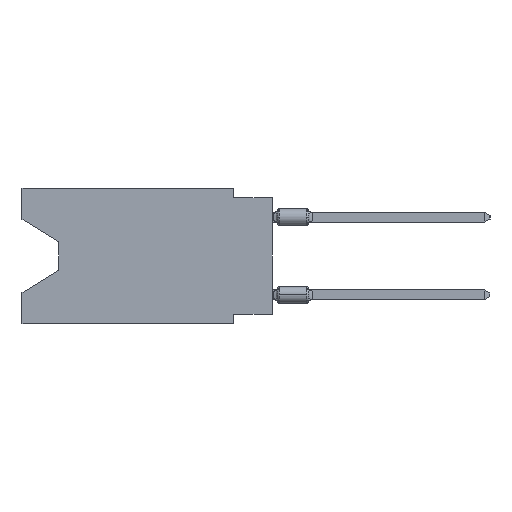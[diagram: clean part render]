
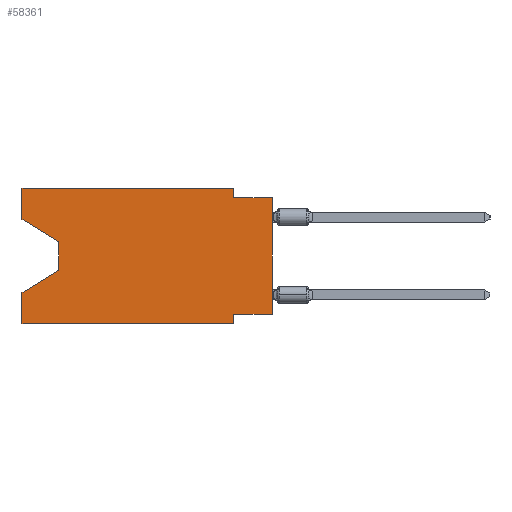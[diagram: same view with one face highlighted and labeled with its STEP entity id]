
A CAD part, left-side view. The second image highlights one B-rep face of the part: STEP entity #58361.
In plain terms, the highlighted planar face has unit normal (-1, 0, 0).
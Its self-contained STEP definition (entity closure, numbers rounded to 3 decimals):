
#2 = CARTESIAN_POINT ( 'NONE',  ( 0., 13.97, -5.385 ) ) ;
#44 = LINE ( 'NONE', #68377, #68410 ) ;
#96 = VERTEX_POINT ( 'NONE', #14504 ) ;
#595 = VERTEX_POINT ( 'NONE', #54141 ) ;
#1430 = ORIENTED_EDGE ( 'NONE', *, *, #9033, .T. ) ;
#1491 = EDGE_CURVE ( 'NONE', #27973, #48108, #33830, .T. ) ;
#1894 = LINE ( 'NONE', #55572, #65405 ) ;
#3446 = EDGE_CURVE ( 'NONE', #29089, #27973, #61913, .T. ) ;
#4562 = VECTOR ( 'NONE', #18804, 1000. ) ;
#4643 = DIRECTION ( 'NONE',  ( 0., 0., -1. ) ) ;
#6801 = CARTESIAN_POINT ( 'NONE',  ( 0., 2.54, 0. ) ) ;
#7218 = CARTESIAN_POINT ( 'NONE',  ( 0., 16.383, -2.038 ) ) ;
#8457 = VECTOR ( 'NONE', #26323, 1000. ) ;
#8740 = CARTESIAN_POINT ( 'NONE',  ( 0., 16.383, -6.852 ) ) ;
#9033 = EDGE_CURVE ( 'NONE', #48108, #32076, #20736, .T. ) ;
#9254 = CARTESIAN_POINT ( 'NONE',  ( 0., 0., -8.255 ) ) ;
#10105 = EDGE_CURVE ( 'NONE', #14759, #96, #62402, .T. ) ;
#11089 = ORIENTED_EDGE ( 'NONE', *, *, #20183, .T. ) ;
#11769 = ORIENTED_EDGE ( 'NONE', *, *, #59760, .F. ) ;
#12449 = DIRECTION ( 'NONE',  ( 0., -1., 0. ) ) ;
#12720 = AXIS2_PLACEMENT_3D ( 'NONE', #62862, #52406, #4643 ) ;
#12785 = CARTESIAN_POINT ( 'NONE',  ( 0., 13.97, -3.505 ) ) ;
#14504 = CARTESIAN_POINT ( 'NONE',  ( 0., 2.54, -8.89 ) ) ;
#14759 = VERTEX_POINT ( 'NONE', #41415 ) ;
#14832 = LINE ( 'NONE', #9254, #31881 ) ;
#18024 = EDGE_LOOP ( 'NONE', ( #64068, #19802, #1430, #45340, #11089, #64749, #50941, #44433, #61040, #11769, #22272, #67755 ) ) ;
#18804 = DIRECTION ( 'NONE',  ( 0., 0., -1. ) ) ;
#19235 = VECTOR ( 'NONE', #25319, 1000. ) ;
#19802 = ORIENTED_EDGE ( 'NONE', *, *, #1491, .T. ) ;
#20183 = EDGE_CURVE ( 'NONE', #51797, #96, #40516, .T. ) ;
#20736 = LINE ( 'NONE', #64302, #8457 ) ;
#20793 = VECTOR ( 'NONE', #41653, 1000. ) ;
#22272 = ORIENTED_EDGE ( 'NONE', *, *, #30496, .F. ) ;
#23642 = LINE ( 'NONE', #30855, #20793 ) ;
#25023 = EDGE_CURVE ( 'NONE', #51797, #32076, #55082, .T. ) ;
#25319 = DIRECTION ( 'NONE',  ( 0., -0.855, -0.519 ) ) ;
#25593 = FACE_OUTER_BOUND ( 'NONE', #18024, .T. ) ;
#26323 = DIRECTION ( 'NONE',  ( 0., 0.855, -0.519 ) ) ;
#26567 = DIRECTION ( 'NONE',  ( 0., 0., 1. ) ) ;
#26668 = VECTOR ( 'NONE', #28956, 1000. ) ;
#27403 = VERTEX_POINT ( 'NONE', #52255 ) ;
#27493 = CARTESIAN_POINT ( 'NONE',  ( 0., 0., -0.635 ) ) ;
#27973 = VERTEX_POINT ( 'NONE', #12785 ) ;
#28956 = DIRECTION ( 'NONE',  ( 0., 0., 1. ) ) ;
#29051 = EDGE_CURVE ( 'NONE', #27403, #51496, #37946, .T. ) ;
#29089 = VERTEX_POINT ( 'NONE', #7218 ) ;
#29853 = DIRECTION ( 'NONE',  ( 0., 1., 0. ) ) ;
#30100 = CARTESIAN_POINT ( 'NONE',  ( 0., 2.54, 0. ) ) ;
#30496 = EDGE_CURVE ( 'NONE', #34547, #38015, #1894, .T. ) ;
#30855 = CARTESIAN_POINT ( 'NONE',  ( 0., 16.383, 0. ) ) ;
#31881 = VECTOR ( 'NONE', #29853, 1000. ) ;
#32076 = VERTEX_POINT ( 'NONE', #8740 ) ;
#33830 = LINE ( 'NONE', #34517, #4562 ) ;
#34517 = CARTESIAN_POINT ( 'NONE',  ( 0., 13.97, -3.505 ) ) ;
#34547 = VERTEX_POINT ( 'NONE', #50335 ) ;
#35319 = EDGE_CURVE ( 'NONE', #595, #14759, #14832, .T. ) ;
#37768 = VECTOR ( 'NONE', #61787, 1000. ) ;
#37946 = LINE ( 'NONE', #27493, #57774 ) ;
#38015 = VERTEX_POINT ( 'NONE', #30100 ) ;
#40516 = LINE ( 'NONE', #66329, #37768 ) ;
#41415 = CARTESIAN_POINT ( 'NONE',  ( 0., 2.54, -8.255 ) ) ;
#41602 = PLANE ( 'NONE',  #12720 ) ;
#41653 = DIRECTION ( 'NONE',  ( 0., 0., 1. ) ) ;
#44433 = ORIENTED_EDGE ( 'NONE', *, *, #59942, .T. ) ;
#45301 = CARTESIAN_POINT ( 'NONE',  ( 0., 16.383, 0. ) ) ;
#45340 = ORIENTED_EDGE ( 'NONE', *, *, #25023, .F. ) ;
#47210 = VECTOR ( 'NONE', #54554, 1000. ) ;
#47427 = CARTESIAN_POINT ( 'NONE',  ( 0., 16.383, -8.89 ) ) ;
#48108 = VERTEX_POINT ( 'NONE', #2 ) ;
#50335 = CARTESIAN_POINT ( 'NONE',  ( 0., 16.383, 0. ) ) ;
#50941 = ORIENTED_EDGE ( 'NONE', *, *, #35319, .F. ) ;
#50961 = LINE ( 'NONE', #6801, #47210 ) ;
#51496 = VERTEX_POINT ( 'NONE', #54580 ) ;
#51797 = VERTEX_POINT ( 'NONE', #47427 ) ;
#52255 = CARTESIAN_POINT ( 'NONE',  ( 0., 2.54, -0.635 ) ) ;
#52281 = DIRECTION ( 'NONE',  ( 0., 0., -1. ) ) ;
#52406 = DIRECTION ( 'NONE',  ( 1., 0., 0. ) ) ;
#54141 = CARTESIAN_POINT ( 'NONE',  ( 0., 0., -8.255 ) ) ;
#54554 = DIRECTION ( 'NONE',  ( 0., 0., -1. ) ) ;
#54580 = CARTESIAN_POINT ( 'NONE',  ( 0., 0., -0.635 ) ) ;
#55082 = LINE ( 'NONE', #45301, #26668 ) ;
#55572 = CARTESIAN_POINT ( 'NONE',  ( 0., 16.383, 0. ) ) ;
#56735 = EDGE_CURVE ( 'NONE', #29089, #34547, #23642, .T. ) ;
#57015 = CARTESIAN_POINT ( 'NONE',  ( 0., 16.383, -2.038 ) ) ;
#57511 = CARTESIAN_POINT ( 'NONE',  ( 0., 2.54, -8.89 ) ) ;
#57774 = VECTOR ( 'NONE', #12449, 1000. ) ;
#58361 = ADVANCED_FACE ( 'NONE', ( #25593 ), #41602, .F. ) ;
#59760 = EDGE_CURVE ( 'NONE', #38015, #27403, #50961, .T. ) ;
#59942 = EDGE_CURVE ( 'NONE', #595, #51496, #44, .T. ) ;
#60482 = DIRECTION ( 'NONE',  ( 0., -1., 0. ) ) ;
#61040 = ORIENTED_EDGE ( 'NONE', *, *, #29051, .F. ) ;
#61787 = DIRECTION ( 'NONE',  ( 0., -1., 0. ) ) ;
#61913 = LINE ( 'NONE', #57015, #19235 ) ;
#62073 = VECTOR ( 'NONE', #52281, 1000. ) ;
#62402 = LINE ( 'NONE', #57511, #62073 ) ;
#62862 = CARTESIAN_POINT ( 'NONE',  ( 0., 16.383, 0. ) ) ;
#64068 = ORIENTED_EDGE ( 'NONE', *, *, #3446, .T. ) ;
#64302 = CARTESIAN_POINT ( 'NONE',  ( 0., 13.97, -5.385 ) ) ;
#64749 = ORIENTED_EDGE ( 'NONE', *, *, #10105, .F. ) ;
#65405 = VECTOR ( 'NONE', #60482, 1000. ) ;
#66329 = CARTESIAN_POINT ( 'NONE',  ( 0., 16.383, -8.89 ) ) ;
#67755 = ORIENTED_EDGE ( 'NONE', *, *, #56735, .F. ) ;
#68377 = CARTESIAN_POINT ( 'NONE',  ( 0., 0., 0. ) ) ;
#68410 = VECTOR ( 'NONE', #26567, 1000. ) ;
